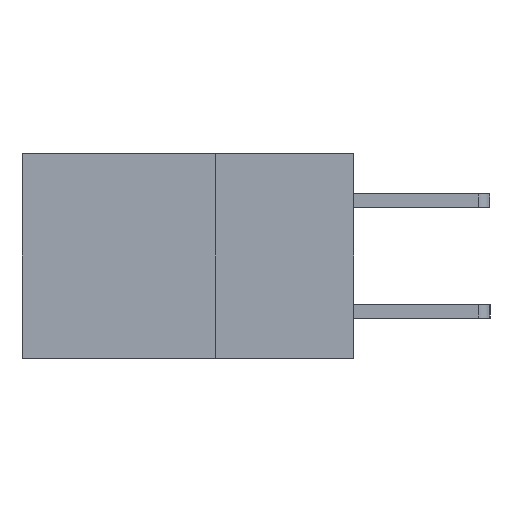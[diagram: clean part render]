
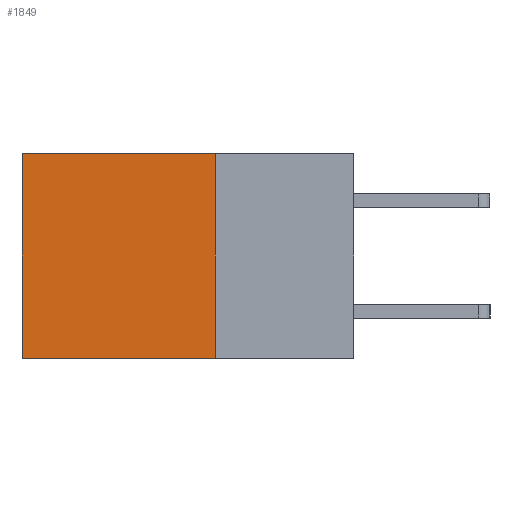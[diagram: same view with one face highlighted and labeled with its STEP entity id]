
A CAD part, left-side view. The second image highlights one B-rep face of the part: STEP entity #1849.
In plain terms, the highlighted planar face has unit normal (-1, 0, 0).
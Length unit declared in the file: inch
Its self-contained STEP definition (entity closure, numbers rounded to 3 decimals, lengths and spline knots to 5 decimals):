
#340 = ORIENTED_EDGE ( 'NONE', *, *, #2830, .F. ) ;
#372 = PLANE ( 'NONE',  #376 ) ;
#376 = AXIS2_PLACEMENT_3D ( 'NONE', #8534, #1934, #468 ) ;
#468 = DIRECTION ( 'NONE',  ( 0., 0., -1. ) ) ;
#601 = DIRECTION ( 'NONE',  ( 0., 0., -1. ) ) ;
#743 = VECTOR ( 'NONE', #5529, 39.37008 ) ;
#868 = ORIENTED_EDGE ( 'NONE', *, *, #7834, .T. ) ;
#1152 = VECTOR ( 'NONE', #1910, 39.37008 ) ;
#1303 = CARTESIAN_POINT ( 'NONE',  ( 0.2875, 0.6, 0. ) ) ;
#1683 = VECTOR ( 'NONE', #601, 39.37008 ) ;
#1849 = ADVANCED_FACE ( 'NONE', ( #5587 ), #372, .F. ) ;
#1910 = DIRECTION ( 'NONE',  ( 0., 1., 0. ) ) ;
#1934 = DIRECTION ( 'NONE',  ( 1., 0., 0. ) ) ;
#2020 = VERTEX_POINT ( 'NONE', #8248 ) ;
#2830 = EDGE_CURVE ( 'NONE', #8807, #6741, #3343, .T. ) ;
#3343 = LINE ( 'NONE', #5559, #1152 ) ;
#4901 = CARTESIAN_POINT ( 'NONE',  ( 0.2875, 0.25, 0. ) ) ;
#4967 = EDGE_LOOP ( 'NONE', ( #8605, #340, #6295, #868 ) ) ;
#5341 = CARTESIAN_POINT ( 'NONE',  ( 0.2875, 0.6, -0.37 ) ) ;
#5529 = DIRECTION ( 'NONE',  ( 0., 0., -1. ) ) ;
#5559 = CARTESIAN_POINT ( 'NONE',  ( 0.2875, 0.25, -0.37 ) ) ;
#5587 = FACE_OUTER_BOUND ( 'NONE', #4967, .T. ) ;
#5594 = CARTESIAN_POINT ( 'NONE',  ( 0.2875, 0.25, 0. ) ) ;
#5622 = VERTEX_POINT ( 'NONE', #8547 ) ;
#6020 = CARTESIAN_POINT ( 'NONE',  ( 0.2875, 0.25, -0.37 ) ) ;
#6247 = EDGE_CURVE ( 'NONE', #2020, #8807, #7765, .T. ) ;
#6295 = ORIENTED_EDGE ( 'NONE', *, *, #6247, .F. ) ;
#6394 = LINE ( 'NONE', #1303, #1683 ) ;
#6741 = VERTEX_POINT ( 'NONE', #5341 ) ;
#7021 = LINE ( 'NONE', #5594, #7846 ) ;
#7765 = LINE ( 'NONE', #4901, #743 ) ;
#7834 = EDGE_CURVE ( 'NONE', #2020, #5622, #7021, .T. ) ;
#7846 = VECTOR ( 'NONE', #8636, 39.37008 ) ;
#8248 = CARTESIAN_POINT ( 'NONE',  ( 0.2875, 0.25, 0. ) ) ;
#8534 = CARTESIAN_POINT ( 'NONE',  ( 0.2875, 0.25, 0. ) ) ;
#8547 = CARTESIAN_POINT ( 'NONE',  ( 0.2875, 0.6, 0. ) ) ;
#8605 = ORIENTED_EDGE ( 'NONE', *, *, #9215, .T. ) ;
#8636 = DIRECTION ( 'NONE',  ( 0., 1., 0. ) ) ;
#8807 = VERTEX_POINT ( 'NONE', #6020 ) ;
#9215 = EDGE_CURVE ( 'NONE', #5622, #6741, #6394, .T. ) ;
